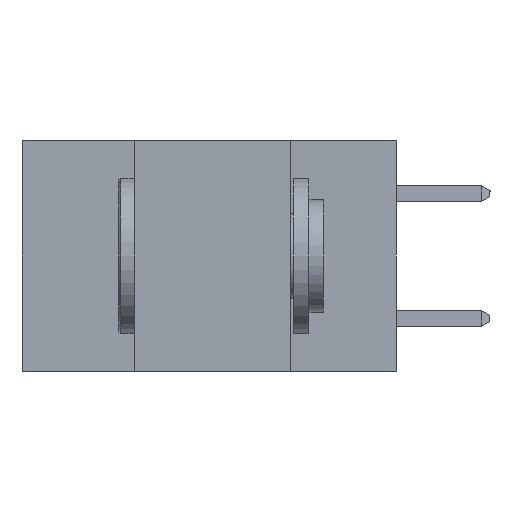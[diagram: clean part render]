
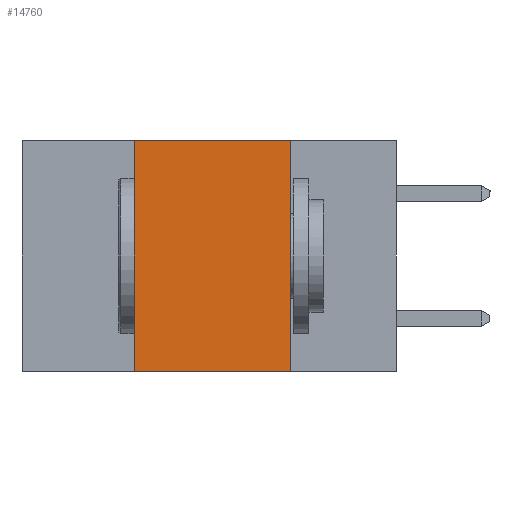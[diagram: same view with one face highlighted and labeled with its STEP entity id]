
A CAD part, left-side view. The second image highlights one B-rep face of the part: STEP entity #14760.
In plain terms, the highlighted planar face has unit normal (-1, 0, 0).
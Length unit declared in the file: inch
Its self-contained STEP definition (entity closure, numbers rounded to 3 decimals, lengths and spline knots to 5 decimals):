
#226 = CARTESIAN_POINT ( 'NONE',  ( 0., 0.6, 0. ) ) ;
#417 = CARTESIAN_POINT ( 'NONE',  ( 0., 0.17, -0.37 ) ) ;
#1421 = LINE ( 'NONE', #9237, #6254 ) ;
#2759 = LINE ( 'NONE', #7944, #10901 ) ;
#4370 = PLANE ( 'NONE',  #11509 ) ;
#4415 = EDGE_CURVE ( 'NONE', #7072, #10124, #14768, .T. ) ;
#4485 = VECTOR ( 'NONE', #12094, 39.37008 ) ;
#4553 = DIRECTION ( 'NONE',  ( 1., 0., 0. ) ) ;
#5725 = CARTESIAN_POINT ( 'NONE',  ( 0., 0.42, 0. ) ) ;
#5754 = ORIENTED_EDGE ( 'NONE', *, *, #10390, .F. ) ;
#6095 = LINE ( 'NONE', #7627, #8407 ) ;
#6254 = VECTOR ( 'NONE', #10566, 39.37008 ) ;
#6683 = CARTESIAN_POINT ( 'NONE',  ( 0., 0.42, -0.37 ) ) ;
#7072 = VERTEX_POINT ( 'NONE', #9461 ) ;
#7627 = CARTESIAN_POINT ( 'NONE',  ( 0., 0.42, -0.37 ) ) ;
#7944 = CARTESIAN_POINT ( 'NONE',  ( 0., 0.6, 0. ) ) ;
#8129 = CARTESIAN_POINT ( 'NONE',  ( 0., 0.17, -0.37 ) ) ;
#8407 = VECTOR ( 'NONE', #12889, 39.37008 ) ;
#9122 = DIRECTION ( 'NONE',  ( 0., -1., 0. ) ) ;
#9237 = CARTESIAN_POINT ( 'NONE',  ( 0., 0.6, -0.37 ) ) ;
#9461 = CARTESIAN_POINT ( 'NONE',  ( 0., 0.17, 0. ) ) ;
#9508 = ORIENTED_EDGE ( 'NONE', *, *, #10672, .T. ) ;
#10124 = VERTEX_POINT ( 'NONE', #417 ) ;
#10390 = EDGE_CURVE ( 'NONE', #15658, #7072, #2759, .T. ) ;
#10566 = DIRECTION ( 'NONE',  ( 0., -1., 0. ) ) ;
#10672 = EDGE_CURVE ( 'NONE', #12902, #10124, #1421, .T. ) ;
#10901 = VECTOR ( 'NONE', #9122, 39.37008 ) ;
#11509 = AXIS2_PLACEMENT_3D ( 'NONE', #226, #4553, #14717 ) ;
#12094 = DIRECTION ( 'NONE',  ( 0., 0., -1. ) ) ;
#12770 = EDGE_CURVE ( 'NONE', #12902, #15658, #6095, .T. ) ;
#12889 = DIRECTION ( 'NONE',  ( 0., 0., 1. ) ) ;
#12902 = VERTEX_POINT ( 'NONE', #6683 ) ;
#13346 = ORIENTED_EDGE ( 'NONE', *, *, #4415, .F. ) ;
#13575 = FACE_OUTER_BOUND ( 'NONE', #15225, .T. ) ;
#13701 = ORIENTED_EDGE ( 'NONE', *, *, #12770, .F. ) ;
#14717 = DIRECTION ( 'NONE',  ( 0., 0., -1. ) ) ;
#14760 = ADVANCED_FACE ( 'NONE', ( #13575 ), #4370, .F. ) ;
#14768 = LINE ( 'NONE', #8129, #4485 ) ;
#15225 = EDGE_LOOP ( 'NONE', ( #13346, #5754, #13701, #9508 ) ) ;
#15658 = VERTEX_POINT ( 'NONE', #5725 ) ;
